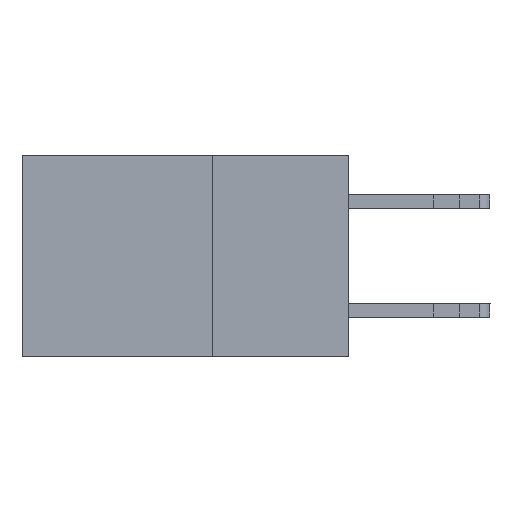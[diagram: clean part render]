
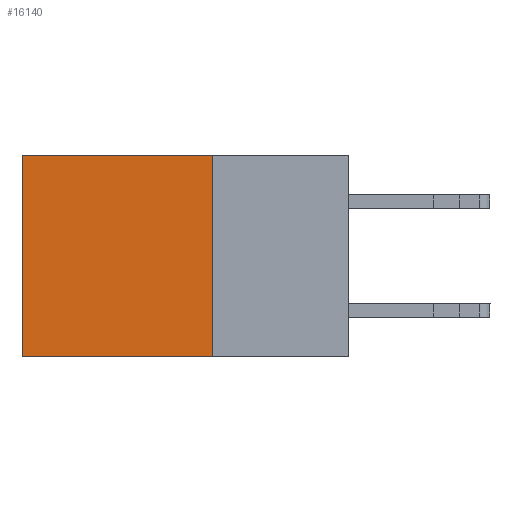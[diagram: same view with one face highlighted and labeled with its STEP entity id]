
A CAD part, left-side view. The second image highlights one B-rep face of the part: STEP entity #16140.
In plain terms, the highlighted planar face has unit normal (-1, 0, 0).
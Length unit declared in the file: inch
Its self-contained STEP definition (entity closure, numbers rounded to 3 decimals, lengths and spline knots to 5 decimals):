
#607 = LINE ( 'NONE', #16087, #7492 ) ;
#1248 = EDGE_CURVE ( 'NONE', #9152, #13612, #607, .T. ) ;
#1637 = LINE ( 'NONE', #1867, #5627 ) ;
#1867 = CARTESIAN_POINT ( 'NONE',  ( 0.2615, 0.25, -0.37 ) ) ;
#2562 = DIRECTION ( 'NONE',  ( 0., 0., -1. ) ) ;
#3036 = ORIENTED_EDGE ( 'NONE', *, *, #13786, .F. ) ;
#3466 = EDGE_CURVE ( 'NONE', #5397, #13612, #1637, .T. ) ;
#3522 = DIRECTION ( 'NONE',  ( 0., 0., -1. ) ) ;
#5139 = CARTESIAN_POINT ( 'NONE',  ( 0.2615, 0.6, 0. ) ) ;
#5397 = VERTEX_POINT ( 'NONE', #16372 ) ;
#5627 = VECTOR ( 'NONE', #20842, 39.37008 ) ;
#5917 = ORIENTED_EDGE ( 'NONE', *, *, #1248, .T. ) ;
#7448 = LINE ( 'NONE', #14914, #15729 ) ;
#7492 = VECTOR ( 'NONE', #2562, 39.37008 ) ;
#7591 = FACE_OUTER_BOUND ( 'NONE', #14002, .T. ) ;
#9152 = VERTEX_POINT ( 'NONE', #5139 ) ;
#9439 = VECTOR ( 'NONE', #10806, 39.37008 ) ;
#10806 = DIRECTION ( 'NONE',  ( 0., 0., -1. ) ) ;
#12390 = VERTEX_POINT ( 'NONE', #14272 ) ;
#13494 = DIRECTION ( 'NONE',  ( 1., 0., 0. ) ) ;
#13612 = VERTEX_POINT ( 'NONE', #17063 ) ;
#13786 = EDGE_CURVE ( 'NONE', #12390, #5397, #18202, .T. ) ;
#14002 = EDGE_LOOP ( 'NONE', ( #5917, #17197, #3036, #19587 ) ) ;
#14209 = CARTESIAN_POINT ( 'NONE',  ( 0.2615, 0.25, -0.37 ) ) ;
#14272 = CARTESIAN_POINT ( 'NONE',  ( 0.2615, 0.25, 0. ) ) ;
#14914 = CARTESIAN_POINT ( 'NONE',  ( 0.2615, 0.25, 0. ) ) ;
#15729 = VECTOR ( 'NONE', #16683, 39.37008 ) ;
#16087 = CARTESIAN_POINT ( 'NONE',  ( 0.2615, 0.6, -0.37 ) ) ;
#16140 = ADVANCED_FACE ( 'NONE', ( #7591 ), #19973, .F. ) ;
#16372 = CARTESIAN_POINT ( 'NONE',  ( 0.2615, 0.25, -0.37 ) ) ;
#16683 = DIRECTION ( 'NONE',  ( 0., 1., 0. ) ) ;
#17028 = AXIS2_PLACEMENT_3D ( 'NONE', #18346, #13494, #3522 ) ;
#17063 = CARTESIAN_POINT ( 'NONE',  ( 0.2615, 0.6, -0.37 ) ) ;
#17197 = ORIENTED_EDGE ( 'NONE', *, *, #3466, .F. ) ;
#18202 = LINE ( 'NONE', #14209, #9439 ) ;
#18346 = CARTESIAN_POINT ( 'NONE',  ( 0.2615, 0.25, -0.37 ) ) ;
#19587 = ORIENTED_EDGE ( 'NONE', *, *, #19904, .T. ) ;
#19904 = EDGE_CURVE ( 'NONE', #12390, #9152, #7448, .T. ) ;
#19973 = PLANE ( 'NONE',  #17028 ) ;
#20842 = DIRECTION ( 'NONE',  ( 0., 1., 0. ) ) ;
